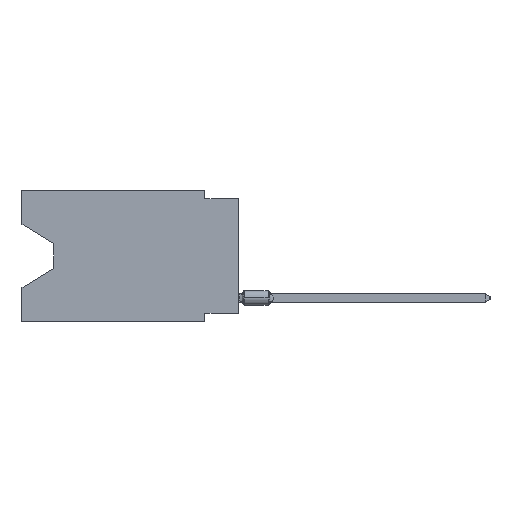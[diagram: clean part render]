
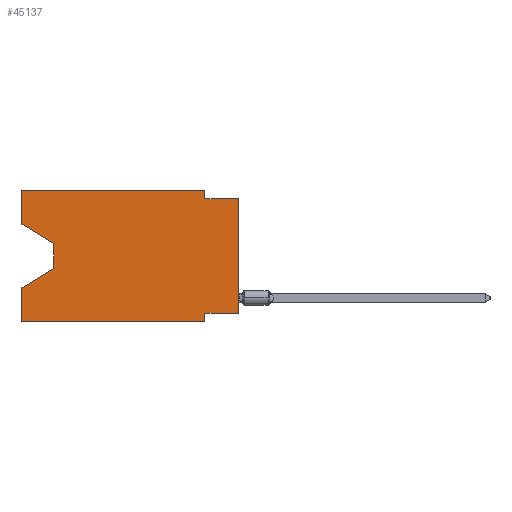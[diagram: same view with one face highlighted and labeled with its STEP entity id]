
A CAD part, left-side view. The second image highlights one B-rep face of the part: STEP entity #45137.
In plain terms, the highlighted planar face has unit normal (-1, 0, 0).
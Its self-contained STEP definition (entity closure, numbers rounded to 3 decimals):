
#441 = DIRECTION ( 'NONE',  ( 0., 0., -1. ) ) ;
#1276 = EDGE_CURVE ( 'NONE', #40724, #34495, #44189, .T. ) ;
#2267 = CARTESIAN_POINT ( 'NONE',  ( 0., 16.383, 0. ) ) ;
#2618 = VERTEX_POINT ( 'NONE', #10666 ) ;
#3103 = VECTOR ( 'NONE', #38034, 1000. ) ;
#3310 = LINE ( 'NONE', #43259, #23214 ) ;
#3349 = VERTEX_POINT ( 'NONE', #38380 ) ;
#3907 = LINE ( 'NONE', #43640, #16906 ) ;
#4813 = CARTESIAN_POINT ( 'NONE',  ( 0., 0., -0.635 ) ) ;
#5896 = CARTESIAN_POINT ( 'NONE',  ( 0., 2.54, -9.906 ) ) ;
#5972 = DIRECTION ( 'NONE',  ( 0., 0., -1. ) ) ;
#6082 = VECTOR ( 'NONE', #14682, 1000. ) ;
#7639 = LINE ( 'NONE', #7889, #35204 ) ;
#7889 = CARTESIAN_POINT ( 'NONE',  ( 0., 0., 0. ) ) ;
#9570 = DIRECTION ( 'NONE',  ( 0., -1., 0. ) ) ;
#10023 = LINE ( 'NONE', #27653, #39576 ) ;
#10421 = ORIENTED_EDGE ( 'NONE', *, *, #28656, .F. ) ;
#10666 = CARTESIAN_POINT ( 'NONE',  ( 0., 0., -0.635 ) ) ;
#12470 = CARTESIAN_POINT ( 'NONE',  ( 0., 2.54, -9.271 ) ) ;
#12532 = CARTESIAN_POINT ( 'NONE',  ( 0., 16.383, -7.36 ) ) ;
#13407 = EDGE_LOOP ( 'NONE', ( #31848, #40014, #16071, #43833, #20354, #10421, #42850, #32355, #37484, #19616, #43134, #35296 ) ) ;
#13872 = VERTEX_POINT ( 'NONE', #36192 ) ;
#13960 = VERTEX_POINT ( 'NONE', #33326 ) ;
#14445 = EDGE_CURVE ( 'NONE', #21146, #29755, #45150, .T. ) ;
#14560 = CARTESIAN_POINT ( 'NONE',  ( 0., 0., -9.271 ) ) ;
#14682 = DIRECTION ( 'NONE',  ( 0., -1., 0. ) ) ;
#15506 = LINE ( 'NONE', #4813, #23373 ) ;
#16071 = ORIENTED_EDGE ( 'NONE', *, *, #23211, .T. ) ;
#16332 = LINE ( 'NONE', #2267, #45768 ) ;
#16906 = VECTOR ( 'NONE', #40297, 1000. ) ;
#17798 = LINE ( 'NONE', #33012, #6082 ) ;
#18790 = CARTESIAN_POINT ( 'NONE',  ( 0., 2.54, 0. ) ) ;
#19251 = CARTESIAN_POINT ( 'NONE',  ( 0., 2.54, 0. ) ) ;
#19487 = DIRECTION ( 'NONE',  ( 0., 1., 0. ) ) ;
#19616 = ORIENTED_EDGE ( 'NONE', *, *, #29309, .F. ) ;
#20354 = ORIENTED_EDGE ( 'NONE', *, *, #42113, .T. ) ;
#20720 = CARTESIAN_POINT ( 'NONE',  ( 0., 16.383, 0. ) ) ;
#21146 = VERTEX_POINT ( 'NONE', #31696 ) ;
#22159 = DIRECTION ( 'NONE',  ( 0., 0., 1. ) ) ;
#23211 = EDGE_CURVE ( 'NONE', #13960, #39675, #45587, .T. ) ;
#23214 = VECTOR ( 'NONE', #35665, 1000. ) ;
#23373 = VECTOR ( 'NONE', #30269, 1000. ) ;
#25531 = CARTESIAN_POINT ( 'NONE',  ( 0., 16.383, -9.906 ) ) ;
#26472 = VECTOR ( 'NONE', #38700, 1000. ) ;
#27653 = CARTESIAN_POINT ( 'NONE',  ( 0., 16.383, -9.906 ) ) ;
#28300 = EDGE_CURVE ( 'NONE', #30506, #39675, #16332, .T. ) ;
#28322 = PLANE ( 'NONE',  #37470 ) ;
#28552 = DIRECTION ( 'NONE',  ( 1., 0., 0. ) ) ;
#28656 = EDGE_CURVE ( 'NONE', #34495, #44235, #3907, .T. ) ;
#29309 = EDGE_CURVE ( 'NONE', #45490, #13872, #39951, .T. ) ;
#29755 = VERTEX_POINT ( 'NONE', #36088 ) ;
#30269 = DIRECTION ( 'NONE',  ( 0., -1., 0. ) ) ;
#30506 = VERTEX_POINT ( 'NONE', #25531 ) ;
#30691 = CARTESIAN_POINT ( 'NONE',  ( 0., 13.97, -4.013 ) ) ;
#31696 = CARTESIAN_POINT ( 'NONE',  ( 0., 16.383, -2.546 ) ) ;
#31848 = ORIENTED_EDGE ( 'NONE', *, *, #14445, .T. ) ;
#32355 = ORIENTED_EDGE ( 'NONE', *, *, #44867, .T. ) ;
#33012 = CARTESIAN_POINT ( 'NONE',  ( 0., 16.383, 0. ) ) ;
#33326 = CARTESIAN_POINT ( 'NONE',  ( 0., 13.97, -5.893 ) ) ;
#33937 = EDGE_CURVE ( 'NONE', #21146, #3349, #3310, .T. ) ;
#34495 = VERTEX_POINT ( 'NONE', #12470 ) ;
#34915 = CARTESIAN_POINT ( 'NONE',  ( 0., 16.383, -2.546 ) ) ;
#35204 = VECTOR ( 'NONE', #22159, 1000. ) ;
#35296 = ORIENTED_EDGE ( 'NONE', *, *, #33937, .F. ) ;
#35665 = DIRECTION ( 'NONE',  ( 0., 0., 1. ) ) ;
#35668 = FACE_OUTER_BOUND ( 'NONE', #13407, .T. ) ;
#36088 = CARTESIAN_POINT ( 'NONE',  ( 0., 13.97, -4.013 ) ) ;
#36192 = CARTESIAN_POINT ( 'NONE',  ( 0., 2.54, -0.635 ) ) ;
#36216 = EDGE_CURVE ( 'NONE', #13872, #2618, #15506, .T. ) ;
#37067 = VECTOR ( 'NONE', #19487, 1000. ) ;
#37470 = AXIS2_PLACEMENT_3D ( 'NONE', #20720, #28552, #5972 ) ;
#37484 = ORIENTED_EDGE ( 'NONE', *, *, #36216, .F. ) ;
#37954 = DIRECTION ( 'NONE',  ( 0., 0., 1. ) ) ;
#38034 = DIRECTION ( 'NONE',  ( 0., 0., -1. ) ) ;
#38255 = VECTOR ( 'NONE', #441, 1000. ) ;
#38380 = CARTESIAN_POINT ( 'NONE',  ( 0., 16.383, 0. ) ) ;
#38700 = DIRECTION ( 'NONE',  ( 0., 0.855, -0.519 ) ) ;
#39543 = VECTOR ( 'NONE', #41809, 1000. ) ;
#39576 = VECTOR ( 'NONE', #9570, 1000. ) ;
#39675 = VERTEX_POINT ( 'NONE', #12532 ) ;
#39951 = LINE ( 'NONE', #18790, #38255 ) ;
#40014 = ORIENTED_EDGE ( 'NONE', *, *, #42403, .T. ) ;
#40297 = DIRECTION ( 'NONE',  ( 0., 0., -1. ) ) ;
#40633 = CARTESIAN_POINT ( 'NONE',  ( 0., 0., -9.271 ) ) ;
#40724 = VERTEX_POINT ( 'NONE', #14560 ) ;
#41508 = EDGE_CURVE ( 'NONE', #3349, #45490, #17798, .T. ) ;
#41809 = DIRECTION ( 'NONE',  ( 0., -0.855, -0.519 ) ) ;
#42113 = EDGE_CURVE ( 'NONE', #30506, #44235, #10023, .T. ) ;
#42403 = EDGE_CURVE ( 'NONE', #29755, #13960, #44704, .T. ) ;
#42850 = ORIENTED_EDGE ( 'NONE', *, *, #1276, .F. ) ;
#43134 = ORIENTED_EDGE ( 'NONE', *, *, #41508, .F. ) ;
#43259 = CARTESIAN_POINT ( 'NONE',  ( 0., 16.383, 0. ) ) ;
#43640 = CARTESIAN_POINT ( 'NONE',  ( 0., 2.54, -9.906 ) ) ;
#43833 = ORIENTED_EDGE ( 'NONE', *, *, #28300, .F. ) ;
#44189 = LINE ( 'NONE', #40633, #37067 ) ;
#44235 = VERTEX_POINT ( 'NONE', #5896 ) ;
#44704 = LINE ( 'NONE', #30691, #3103 ) ;
#44867 = EDGE_CURVE ( 'NONE', #40724, #2618, #7639, .T. ) ;
#45137 = ADVANCED_FACE ( 'NONE', ( #35668 ), #28322, .F. ) ;
#45150 = LINE ( 'NONE', #34915, #39543 ) ;
#45490 = VERTEX_POINT ( 'NONE', #19251 ) ;
#45587 = LINE ( 'NONE', #45831, #26472 ) ;
#45768 = VECTOR ( 'NONE', #37954, 1000. ) ;
#45831 = CARTESIAN_POINT ( 'NONE',  ( 0., 13.97, -5.893 ) ) ;
